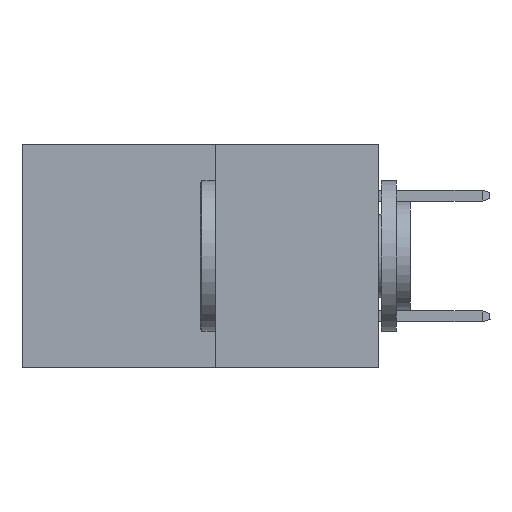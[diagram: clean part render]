
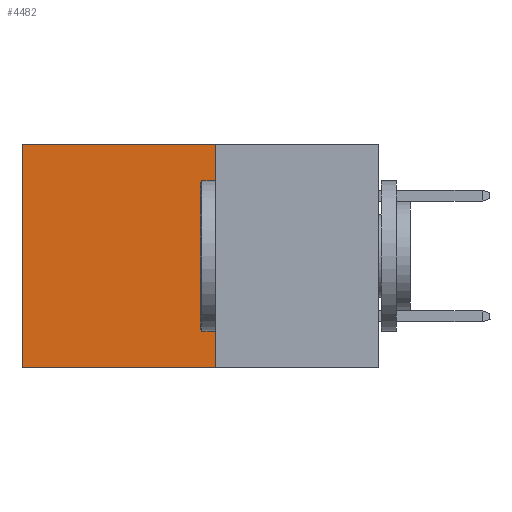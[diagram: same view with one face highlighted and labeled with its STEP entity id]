
A CAD part, left-side view. The second image highlights one B-rep face of the part: STEP entity #4482.
In plain terms, the highlighted planar face has unit normal (-1, 0, 0).
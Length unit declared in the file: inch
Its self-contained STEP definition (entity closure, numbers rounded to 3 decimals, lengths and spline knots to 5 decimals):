
#393 = CARTESIAN_POINT ( 'NONE',  ( 0.277, 0.27, -0.37 ) ) ;
#1351 = EDGE_CURVE ( 'NONE', #8239, #12953, #12534, .T. ) ;
#3496 = EDGE_CURVE ( 'NONE', #8629, #17177, #8070, .T. ) ;
#4482 = ADVANCED_FACE ( 'NONE', ( #6909 ), #14766, .F. ) ;
#4968 = EDGE_CURVE ( 'NONE', #8629, #8239, #6645, .T. ) ;
#5066 = DIRECTION ( 'NONE',  ( 0., 0., -1. ) ) ;
#5134 = DIRECTION ( 'NONE',  ( 1., 0., 0. ) ) ;
#5395 = CARTESIAN_POINT ( 'NONE',  ( 0.277, 0.59, -0.37 ) ) ;
#5636 = AXIS2_PLACEMENT_3D ( 'NONE', #14559, #5134, #5066 ) ;
#6645 = LINE ( 'NONE', #21700, #20402 ) ;
#6909 = FACE_OUTER_BOUND ( 'NONE', #14953, .T. ) ;
#7357 = VECTOR ( 'NONE', #17647, 39.37008 ) ;
#8070 = LINE ( 'NONE', #19383, #20702 ) ;
#8239 = VERTEX_POINT ( 'NONE', #21530 ) ;
#8629 = VERTEX_POINT ( 'NONE', #14131 ) ;
#11326 = ORIENTED_EDGE ( 'NONE', *, *, #4968, .T. ) ;
#12056 = CARTESIAN_POINT ( 'NONE',  ( 0.277, 0.27, -0.37 ) ) ;
#12339 = ORIENTED_EDGE ( 'NONE', *, *, #3496, .F. ) ;
#12534 = LINE ( 'NONE', #22437, #7357 ) ;
#12953 = VERTEX_POINT ( 'NONE', #5395 ) ;
#14131 = CARTESIAN_POINT ( 'NONE',  ( 0.277, 0.27, 0. ) ) ;
#14559 = CARTESIAN_POINT ( 'NONE',  ( 0.277, 0.27, -0.37 ) ) ;
#14722 = ORIENTED_EDGE ( 'NONE', *, *, #16360, .F. ) ;
#14766 = PLANE ( 'NONE',  #5636 ) ;
#14953 = EDGE_LOOP ( 'NONE', ( #20065, #14722, #12339, #11326 ) ) ;
#16360 = EDGE_CURVE ( 'NONE', #17177, #12953, #18062, .T. ) ;
#17177 = VERTEX_POINT ( 'NONE', #393 ) ;
#17647 = DIRECTION ( 'NONE',  ( 0., 0., -1. ) ) ;
#18062 = LINE ( 'NONE', #12056, #22065 ) ;
#19383 = CARTESIAN_POINT ( 'NONE',  ( 0.277, 0.27, -0.37 ) ) ;
#19442 = DIRECTION ( 'NONE',  ( 0., 0., -1. ) ) ;
#20065 = ORIENTED_EDGE ( 'NONE', *, *, #1351, .T. ) ;
#20402 = VECTOR ( 'NONE', #21706, 39.37008 ) ;
#20582 = DIRECTION ( 'NONE',  ( 0., 1., 0. ) ) ;
#20702 = VECTOR ( 'NONE', #19442, 39.37008 ) ;
#21530 = CARTESIAN_POINT ( 'NONE',  ( 0.277, 0.59, 0. ) ) ;
#21700 = CARTESIAN_POINT ( 'NONE',  ( 0.277, 0.27, 0. ) ) ;
#21706 = DIRECTION ( 'NONE',  ( 0., 1., 0. ) ) ;
#22065 = VECTOR ( 'NONE', #20582, 39.37008 ) ;
#22437 = CARTESIAN_POINT ( 'NONE',  ( 0.277, 0.59, -0.37 ) ) ;
